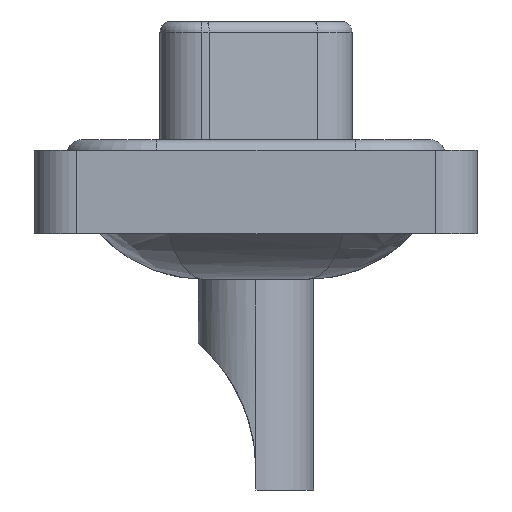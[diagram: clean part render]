
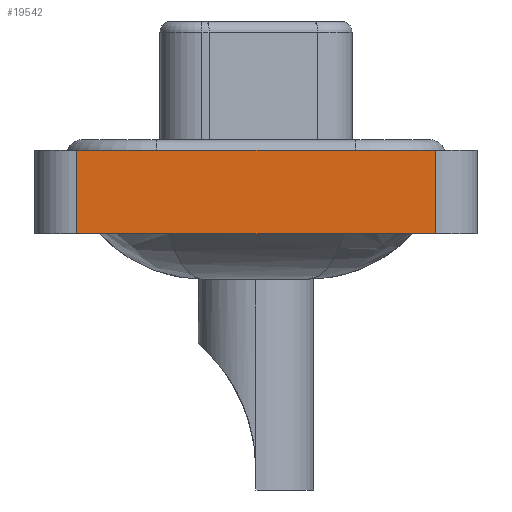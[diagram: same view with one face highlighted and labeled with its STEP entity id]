
A CAD part, left-side view. The second image highlights one B-rep face of the part: STEP entity #19542.
In plain terms, the highlighted planar face has unit normal (-1, 0, 0).
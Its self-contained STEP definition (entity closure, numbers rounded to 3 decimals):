
#208 = VECTOR ( 'NONE', #15273, 1000. ) ;
#493 = VERTEX_POINT ( 'NONE', #4096 ) ;
#548 = DIRECTION ( 'NONE',  ( 0., 0., 1. ) ) ;
#929 = LINE ( 'NONE', #13750, #208 ) ;
#1440 = EDGE_LOOP ( 'NONE', ( #12663, #17931, #7115, #6411 ) ) ;
#1448 = DIRECTION ( 'NONE',  ( 0., -1., 0. ) ) ;
#2186 = DIRECTION ( 'NONE',  ( 0., 0., 1. ) ) ;
#2279 = VERTEX_POINT ( 'NONE', #14787 ) ;
#2340 = FACE_OUTER_BOUND ( 'NONE', #1440, .T. ) ;
#4096 = CARTESIAN_POINT ( 'NONE',  ( -7.35, 8.55, 0.4 ) ) ;
#4183 = LINE ( 'NONE', #18616, #6714 ) ;
#4862 = LINE ( 'NONE', #12036, #21792 ) ;
#5968 = DIRECTION ( 'NONE',  ( -1., 0., 0. ) ) ;
#6411 = ORIENTED_EDGE ( 'NONE', *, *, #23017, .T. ) ;
#6714 = VECTOR ( 'NONE', #2186, 1000. ) ;
#7115 = ORIENTED_EDGE ( 'NONE', *, *, #9159, .F. ) ;
#7356 = EDGE_CURVE ( 'NONE', #493, #14160, #929, .T. ) ;
#7455 = CARTESIAN_POINT ( 'NONE',  ( -7.35, -8.55, -3.6 ) ) ;
#7539 = DIRECTION ( 'NONE',  ( 0., 0., 1. ) ) ;
#9159 = EDGE_CURVE ( 'NONE', #2279, #493, #9633, .T. ) ;
#9498 = PLANE ( 'NONE',  #12030 ) ;
#9633 = LINE ( 'NONE', #12846, #9979 ) ;
#9979 = VECTOR ( 'NONE', #7539, 1000. ) ;
#10219 = CARTESIAN_POINT ( 'NONE',  ( -7.35, -8.55, 0.4 ) ) ;
#12030 = AXIS2_PLACEMENT_3D ( 'NONE', #18203, #5968, #548 ) ;
#12036 = CARTESIAN_POINT ( 'NONE',  ( -7.35, -8.55, -3.6 ) ) ;
#12663 = ORIENTED_EDGE ( 'NONE', *, *, #15016, .T. ) ;
#12846 = CARTESIAN_POINT ( 'NONE',  ( -7.35, 8.55, -3.6 ) ) ;
#13750 = CARTESIAN_POINT ( 'NONE',  ( -7.35, -8.55, 0.4 ) ) ;
#14160 = VERTEX_POINT ( 'NONE', #10219 ) ;
#14787 = CARTESIAN_POINT ( 'NONE',  ( -7.35, 8.55, -3.6 ) ) ;
#15016 = EDGE_CURVE ( 'NONE', #22628, #14160, #4183, .T. ) ;
#15273 = DIRECTION ( 'NONE',  ( 0., -1., 0. ) ) ;
#17931 = ORIENTED_EDGE ( 'NONE', *, *, #7356, .F. ) ;
#18203 = CARTESIAN_POINT ( 'NONE',  ( -7.35, -8.55, -3.6 ) ) ;
#18616 = CARTESIAN_POINT ( 'NONE',  ( -7.35, -8.55, -3.6 ) ) ;
#19542 = ADVANCED_FACE ( 'NONE', ( #2340 ), #9498, .T. ) ;
#21792 = VECTOR ( 'NONE', #1448, 1000. ) ;
#22628 = VERTEX_POINT ( 'NONE', #7455 ) ;
#23017 = EDGE_CURVE ( 'NONE', #2279, #22628, #4862, .T. ) ;
